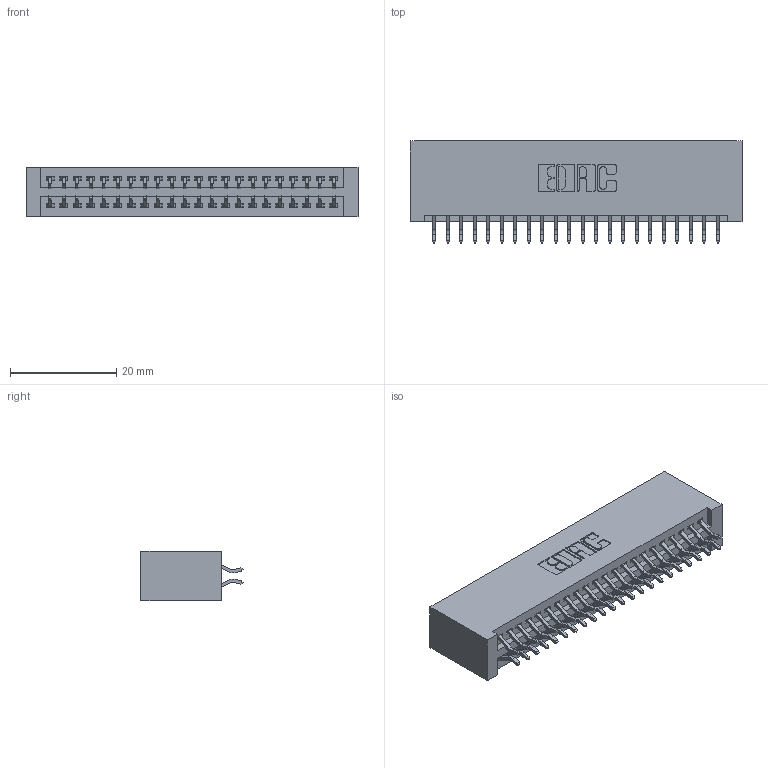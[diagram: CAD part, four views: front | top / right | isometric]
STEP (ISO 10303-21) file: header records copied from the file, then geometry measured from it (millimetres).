
FILE_DESCRIPTION (( 'STEP AP203' ), '1' );
FILE_NAME ('395-044-556-201.STEP', '2018-11-15T21:58:14', ( '' ), ( '' ), 'SwSTEP 2.0', 'SolidWorks 2016', '' );
FILE_SCHEMA (( 'CONFIG_CONTROL_DESIGN' ));
Length unit declared in the file: inch
Products named in the file (3): 345 Part_No Mounting Lugs; 345-292-001_556 Tail; 395-044-556-201
Assembly tree (45 placements, depth 2):
  395-044-556-201
    345 Part_No Mounting Lugs
    345-292-001_556 Tail  x44
Bounding box: 62.48 x 19.24 x 9.4 mm (x, y, z)
Volume: 6498.3 mm3; surface area: 9482.9 mm2
Topology: 45 solids, 45 shells, 2582 faces, 7665 edges, 5050 vertices
Faces by surface type: plane 1704, cylinder 878
Entity records: 19897 total; most frequent: CARTESIAN_POINT 3368, ORIENTED_EDGE 3290, DIRECTION 2977, EDGE_CURVE 1645, LINE 1425, VECTOR 1425, VERTEX_POINT 1094, AXIS2_PLACEMENT_3D 776
